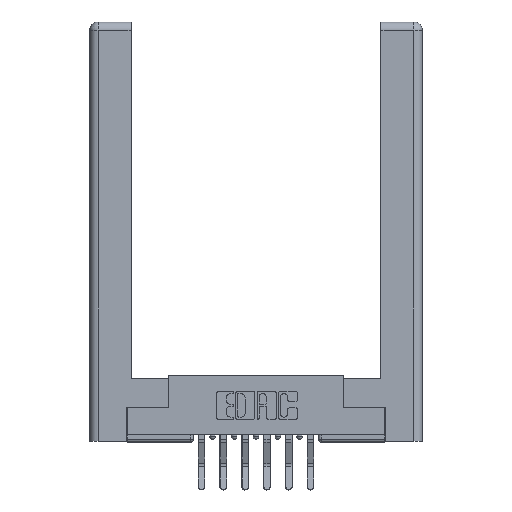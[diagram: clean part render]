
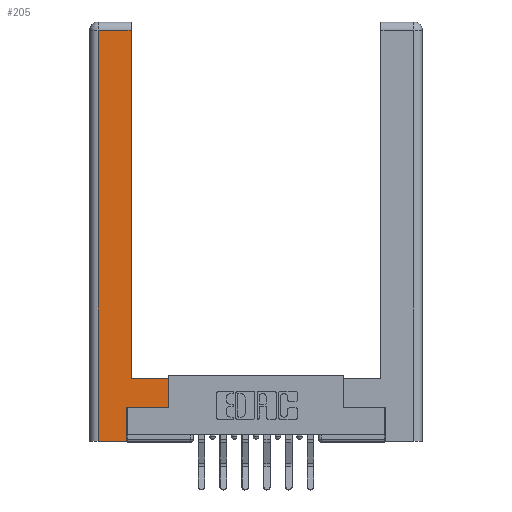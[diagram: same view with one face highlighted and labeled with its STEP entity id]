
A CAD part, top view. The second image highlights one B-rep face of the part: STEP entity #205.
In plain terms, the highlighted planar face has unit normal (0, 0, 1).
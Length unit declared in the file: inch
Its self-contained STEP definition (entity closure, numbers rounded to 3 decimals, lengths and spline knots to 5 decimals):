
#205 = ADVANCED_FACE ( 'NONE', ( #1843 ), #6011, .F. ) ;
#454 = ORIENTED_EDGE ( 'NONE', *, *, #4200, .T. ) ;
#584 = VECTOR ( 'NONE', #3480, 39.37008 ) ;
#618 = CARTESIAN_POINT ( 'NONE',  ( 0.265, 0.245, 0. ) ) ;
#934 = DIRECTION ( 'NONE',  ( 0., -1., 0. ) ) ;
#1114 = DIRECTION ( 'NONE',  ( 1., 0., 0. ) ) ;
#1196 = VECTOR ( 'NONE', #1114, 39.37008 ) ;
#1400 = VECTOR ( 'NONE', #2449, 39.37008 ) ;
#1435 = ORIENTED_EDGE ( 'NONE', *, *, #2279, .T. ) ;
#1843 = FACE_OUTER_BOUND ( 'NONE', #5368, .T. ) ;
#1909 = DIRECTION ( 'NONE',  ( -1., 0., 0. ) ) ;
#2236 = DIRECTION ( 'NONE',  ( 1., 0., 0. ) ) ;
#2260 = ORIENTED_EDGE ( 'NONE', *, *, #9429, .T. ) ;
#2279 = EDGE_CURVE ( 'NONE', #8849, #2907, #10875, .T. ) ;
#2316 = LINE ( 'NONE', #6270, #1400 ) ;
#2401 = LINE ( 'NONE', #4937, #12379 ) ;
#2449 = DIRECTION ( 'NONE',  ( 0., 1., 0. ) ) ;
#2907 = VERTEX_POINT ( 'NONE', #6394 ) ;
#2926 = VERTEX_POINT ( 'NONE', #618 ) ;
#3480 = DIRECTION ( 'NONE',  ( 0., 1., 0. ) ) ;
#3802 = LINE ( 'NONE', #5168, #4580 ) ;
#3883 = VERTEX_POINT ( 'NONE', #9160 ) ;
#4086 = CARTESIAN_POINT ( 'NONE',  ( 0.565, 0.245, 0. ) ) ;
#4195 = VERTEX_POINT ( 'NONE', #12428 ) ;
#4200 = EDGE_CURVE ( 'NONE', #12432, #4195, #5713, .T. ) ;
#4503 = ORIENTED_EDGE ( 'NONE', *, *, #9482, .T. ) ;
#4580 = VECTOR ( 'NONE', #8034, 39.37008 ) ;
#4601 = VECTOR ( 'NONE', #2236, 39.37008 ) ;
#4821 = DIRECTION ( 'NONE',  ( 0., 1., 0. ) ) ;
#4937 = CARTESIAN_POINT ( 'NONE',  ( 0.265, 0.245, 0. ) ) ;
#5126 = VECTOR ( 'NONE', #934, 39.37008 ) ;
#5133 = CARTESIAN_POINT ( 'NONE',  ( 0.0615, 0., 0. ) ) ;
#5168 = CARTESIAN_POINT ( 'NONE',  ( 0.295, 0.45, 0. ) ) ;
#5188 = LINE ( 'NONE', #7844, #4601 ) ;
#5368 = EDGE_LOOP ( 'NONE', ( #11314, #454, #2260, #10140, #12359, #4503, #1435, #10869 ) ) ;
#5621 = VERTEX_POINT ( 'NONE', #9939 ) ;
#5713 = LINE ( 'NONE', #9543, #11622 ) ;
#6011 = PLANE ( 'NONE',  #12150 ) ;
#6019 = LINE ( 'NONE', #11681, #1196 ) ;
#6270 = CARTESIAN_POINT ( 'NONE',  ( 0.295, 3., 0. ) ) ;
#6321 = LINE ( 'NONE', #12533, #5126 ) ;
#6394 = CARTESIAN_POINT ( 'NONE',  ( 0.565, 0.45, 0. ) ) ;
#6640 = DIRECTION ( 'NONE',  ( -1., 0., 0. ) ) ;
#7088 = EDGE_CURVE ( 'NONE', #10499, #5621, #5188, .T. ) ;
#7772 = EDGE_CURVE ( 'NONE', #2907, #3883, #3802, .T. ) ;
#7844 = CARTESIAN_POINT ( 'NONE',  ( 0.265, 0., 0. ) ) ;
#8034 = DIRECTION ( 'NONE',  ( -1., 0., 0. ) ) ;
#8248 = CARTESIAN_POINT ( 'NONE',  ( 0., 0., 0. ) ) ;
#8326 = DIRECTION ( 'NONE',  ( 0., 0., -1. ) ) ;
#8849 = VERTEX_POINT ( 'NONE', #4086 ) ;
#9160 = CARTESIAN_POINT ( 'NONE',  ( 0.295, 0.45, 0. ) ) ;
#9429 = EDGE_CURVE ( 'NONE', #4195, #10499, #6321, .T. ) ;
#9482 = EDGE_CURVE ( 'NONE', #2926, #8849, #6019, .T. ) ;
#9543 = CARTESIAN_POINT ( 'NONE',  ( 0.0615, 2.94, 0. ) ) ;
#9683 = EDGE_CURVE ( 'NONE', #5621, #2926, #2401, .T. ) ;
#9939 = CARTESIAN_POINT ( 'NONE',  ( 0.265, 0., 0. ) ) ;
#10140 = ORIENTED_EDGE ( 'NONE', *, *, #7088, .T. ) ;
#10499 = VERTEX_POINT ( 'NONE', #5133 ) ;
#10869 = ORIENTED_EDGE ( 'NONE', *, *, #7772, .T. ) ;
#10875 = LINE ( 'NONE', #11180, #584 ) ;
#11154 = CARTESIAN_POINT ( 'NONE',  ( 0.295, 2.94, 0. ) ) ;
#11180 = CARTESIAN_POINT ( 'NONE',  ( 0.565, 0.45, 0. ) ) ;
#11314 = ORIENTED_EDGE ( 'NONE', *, *, #11811, .T. ) ;
#11622 = VECTOR ( 'NONE', #1909, 39.37008 ) ;
#11681 = CARTESIAN_POINT ( 'NONE',  ( 0.565, 0.245, 0. ) ) ;
#11811 = EDGE_CURVE ( 'NONE', #3883, #12432, #2316, .T. ) ;
#12150 = AXIS2_PLACEMENT_3D ( 'NONE', #8248, #8326, #6640 ) ;
#12359 = ORIENTED_EDGE ( 'NONE', *, *, #9683, .T. ) ;
#12379 = VECTOR ( 'NONE', #4821, 39.37008 ) ;
#12428 = CARTESIAN_POINT ( 'NONE',  ( 0.0615, 2.94, 0. ) ) ;
#12432 = VERTEX_POINT ( 'NONE', #11154 ) ;
#12533 = CARTESIAN_POINT ( 'NONE',  ( 0.0615, 0., 0. ) ) ;
